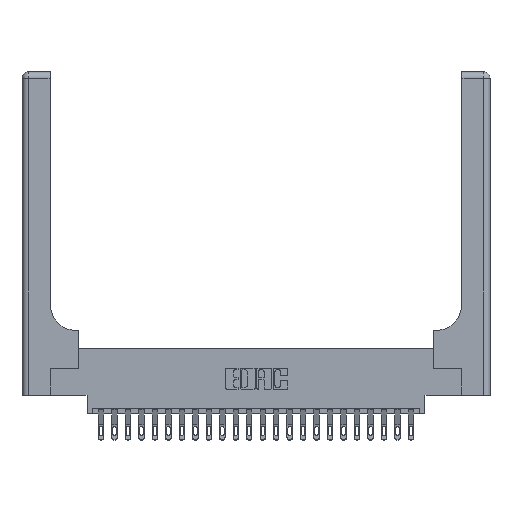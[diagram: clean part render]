
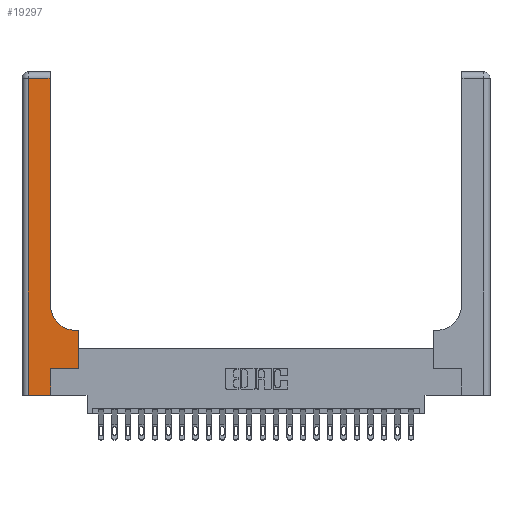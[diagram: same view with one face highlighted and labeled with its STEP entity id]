
A CAD part, top view. The second image highlights one B-rep face of the part: STEP entity #19297.
In plain terms, the highlighted planar face has unit normal (0, 0, 1).
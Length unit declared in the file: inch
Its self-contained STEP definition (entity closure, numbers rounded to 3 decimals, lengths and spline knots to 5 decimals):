
#48 = VERTEX_POINT ( 'NONE', #10668 ) ;
#427 = EDGE_CURVE ( 'NONE', #6012, #18811, #1219, .T. ) ;
#929 = CARTESIAN_POINT ( 'NONE',  ( 0.51, 0.6, 0.37 ) ) ;
#1219 = LINE ( 'NONE', #15802, #21719 ) ;
#1925 = PLANE ( 'NONE',  #3742 ) ;
#1941 = EDGE_CURVE ( 'NONE', #21575, #48, #18356, .T. ) ;
#2724 = ORIENTED_EDGE ( 'NONE', *, *, #10150, .T. ) ;
#2934 = VECTOR ( 'NONE', #20529, 39.37008 ) ;
#3188 = VERTEX_POINT ( 'NONE', #22486 ) ;
#3249 = EDGE_CURVE ( 'NONE', #19506, #12707, #20664, .T. ) ;
#3688 = LINE ( 'NONE', #11023, #5840 ) ;
#3742 = AXIS2_PLACEMENT_3D ( 'NONE', #16642, #15026, #5720 ) ;
#3779 = FACE_OUTER_BOUND ( 'NONE', #23166, .T. ) ;
#5220 = LINE ( 'NONE', #21989, #2934 ) ;
#5720 = DIRECTION ( 'NONE',  ( -1., 0., 0. ) ) ;
#5840 = VECTOR ( 'NONE', #9187, 39.37008 ) ;
#5942 = CIRCLE ( 'NONE', #20808, 0.25 ) ;
#6012 = VERTEX_POINT ( 'NONE', #18880 ) ;
#6192 = CARTESIAN_POINT ( 'NONE',  ( 0.265, 0.25, 0.37 ) ) ;
#7192 = DIRECTION ( 'NONE',  ( -1., 0., 0. ) ) ;
#7694 = DIRECTION ( 'NONE',  ( 0., 1., 0. ) ) ;
#7998 = CARTESIAN_POINT ( 'NONE',  ( 0.265, 0., 0.37 ) ) ;
#8607 = CARTESIAN_POINT ( 'NONE',  ( 0.528, 0.25, 0.37 ) ) ;
#8766 = VERTEX_POINT ( 'NONE', #21945 ) ;
#9027 = DIRECTION ( 'NONE',  ( 0., -1., 0. ) ) ;
#9070 = EDGE_CURVE ( 'NONE', #12707, #21575, #21538, .T. ) ;
#9187 = DIRECTION ( 'NONE',  ( 1., 0., 0. ) ) ;
#9643 = CARTESIAN_POINT ( 'NONE',  ( 0.51, 0.85, 0.37 ) ) ;
#9729 = VECTOR ( 'NONE', #7192, 39.37008 ) ;
#10150 = EDGE_CURVE ( 'NONE', #3188, #8766, #22931, .T. ) ;
#10315 = EDGE_CURVE ( 'NONE', #48, #3188, #3688, .T. ) ;
#10386 = ORIENTED_EDGE ( 'NONE', *, *, #10315, .T. ) ;
#10668 = CARTESIAN_POINT ( 'NONE',  ( 0.06, 0., 0.37 ) ) ;
#10797 = ORIENTED_EDGE ( 'NONE', *, *, #20901, .T. ) ;
#10823 = VECTOR ( 'NONE', #9027, 39.37008 ) ;
#10996 = CARTESIAN_POINT ( 'NONE',  ( 0.06, 3., 0.37 ) ) ;
#11023 = CARTESIAN_POINT ( 'NONE',  ( 0., 0., 0.37 ) ) ;
#12707 = VERTEX_POINT ( 'NONE', #12759 ) ;
#12759 = CARTESIAN_POINT ( 'NONE',  ( 0.26, 2.94, 0.37 ) ) ;
#12910 = VECTOR ( 'NONE', #20986, 39.37008 ) ;
#13064 = DIRECTION ( 'NONE',  ( 1., 0., 0. ) ) ;
#13382 = VECTOR ( 'NONE', #7694, 39.37008 ) ;
#14324 = DIRECTION ( 'NONE',  ( -1., 0., 0. ) ) ;
#14803 = ORIENTED_EDGE ( 'NONE', *, *, #18533, .T. ) ;
#15026 = DIRECTION ( 'NONE',  ( 0., 0., -1. ) ) ;
#15802 = CARTESIAN_POINT ( 'NONE',  ( 0.26, 0.6, 0.37 ) ) ;
#16130 = ORIENTED_EDGE ( 'NONE', *, *, #23422, .T. ) ;
#16505 = CARTESIAN_POINT ( 'NONE',  ( 0., 2.94, 0.37 ) ) ;
#16642 = CARTESIAN_POINT ( 'NONE',  ( 0., 3., 0.37 ) ) ;
#17093 = ORIENTED_EDGE ( 'NONE', *, *, #3249, .T. ) ;
#18154 = CARTESIAN_POINT ( 'NONE',  ( 0.06, 2.94, 0.37 ) ) ;
#18356 = LINE ( 'NONE', #10996, #10823 ) ;
#18533 = EDGE_CURVE ( 'NONE', #24163, #6012, #5220, .T. ) ;
#18811 = VERTEX_POINT ( 'NONE', #929 ) ;
#18817 = DIRECTION ( 'NONE',  ( 0., 0., -1. ) ) ;
#18821 = CARTESIAN_POINT ( 'NONE',  ( 0.26, 3., 0.37 ) ) ;
#18880 = CARTESIAN_POINT ( 'NONE',  ( 0.528, 0.6, 0.37 ) ) ;
#19297 = ADVANCED_FACE ( 'NONE', ( #3779 ), #1925, .F. ) ;
#19506 = VERTEX_POINT ( 'NONE', #21273 ) ;
#20317 = ORIENTED_EDGE ( 'NONE', *, *, #427, .T. ) ;
#20529 = DIRECTION ( 'NONE',  ( 0., 1., 0. ) ) ;
#20664 = LINE ( 'NONE', #18821, #13382 ) ;
#20808 = AXIS2_PLACEMENT_3D ( 'NONE', #9643, #18817, #13064 ) ;
#20901 = EDGE_CURVE ( 'NONE', #8766, #24163, #21252, .T. ) ;
#20986 = DIRECTION ( 'NONE',  ( 0., 1., 0. ) ) ;
#21252 = LINE ( 'NONE', #6192, #23266 ) ;
#21273 = CARTESIAN_POINT ( 'NONE',  ( 0.26, 0.85, 0.37 ) ) ;
#21538 = LINE ( 'NONE', #16505, #9729 ) ;
#21575 = VERTEX_POINT ( 'NONE', #18154 ) ;
#21576 = ORIENTED_EDGE ( 'NONE', *, *, #9070, .T. ) ;
#21719 = VECTOR ( 'NONE', #14324, 39.37008 ) ;
#21945 = CARTESIAN_POINT ( 'NONE',  ( 0.265, 0.25, 0.37 ) ) ;
#21989 = CARTESIAN_POINT ( 'NONE',  ( 0.528, 0.25, 0.37 ) ) ;
#22486 = CARTESIAN_POINT ( 'NONE',  ( 0.265, 0., 0.37 ) ) ;
#22931 = LINE ( 'NONE', #7998, #12910 ) ;
#22963 = DIRECTION ( 'NONE',  ( 1., 0., 0. ) ) ;
#23166 = EDGE_LOOP ( 'NONE', ( #17093, #21576, #23994, #10386, #2724, #10797, #14803, #20317, #16130 ) ) ;
#23266 = VECTOR ( 'NONE', #22963, 39.37008 ) ;
#23422 = EDGE_CURVE ( 'NONE', #18811, #19506, #5942, .T. ) ;
#23994 = ORIENTED_EDGE ( 'NONE', *, *, #1941, .T. ) ;
#24163 = VERTEX_POINT ( 'NONE', #8607 ) ;
